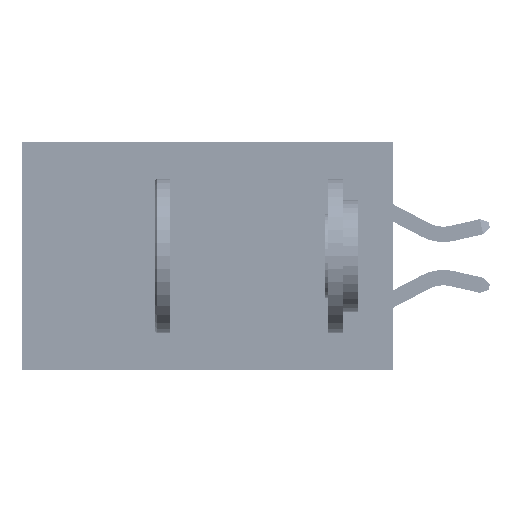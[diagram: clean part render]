
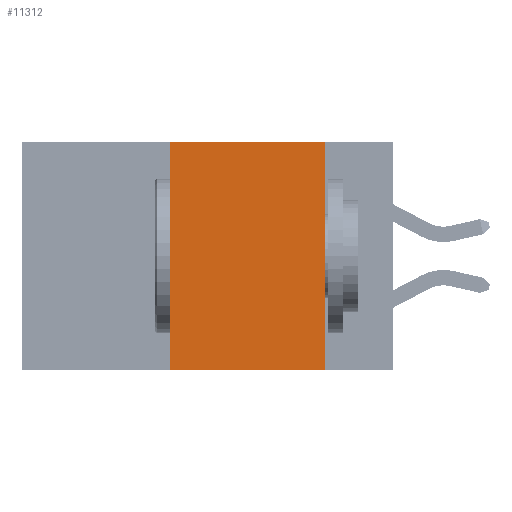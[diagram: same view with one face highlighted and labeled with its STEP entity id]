
A CAD part, left-side view. The second image highlights one B-rep face of the part: STEP entity #11312.
In plain terms, the highlighted planar face has unit normal (-1, 0, 0).
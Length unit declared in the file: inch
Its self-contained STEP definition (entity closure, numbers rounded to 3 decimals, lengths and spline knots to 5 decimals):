
#204 = FACE_OUTER_BOUND ( 'NONE', #42144, .T. ) ;
#1945 = VERTEX_POINT ( 'NONE', #15128 ) ;
#3687 = EDGE_CURVE ( 'NONE', #16818, #43986, #29375, .T. ) ;
#4079 = DIRECTION ( 'NONE',  ( 1., 0., 0. ) ) ;
#8083 = AXIS2_PLACEMENT_3D ( 'NONE', #42821, #4079, #28879 ) ;
#8617 = VECTOR ( 'NONE', #16722, 39.37008 ) ;
#10317 = DIRECTION ( 'NONE',  ( 0., 0., 1. ) ) ;
#11312 = ADVANCED_FACE ( 'NONE', ( #204 ), #25348, .F. ) ;
#11529 = ORIENTED_EDGE ( 'NONE', *, *, #35160, .T. ) ;
#12072 = CARTESIAN_POINT ( 'NONE',  ( 0., 0.36, 0. ) ) ;
#12078 = LINE ( 'NONE', #41416, #39032 ) ;
#15128 = CARTESIAN_POINT ( 'NONE',  ( 0., 0.36, -0.37 ) ) ;
#16722 = DIRECTION ( 'NONE',  ( 0., -1., 0. ) ) ;
#16818 = VERTEX_POINT ( 'NONE', #12072 ) ;
#20365 = DIRECTION ( 'NONE',  ( 0., 0., -1. ) ) ;
#21157 = DIRECTION ( 'NONE',  ( 0., -1., 0. ) ) ;
#23649 = CARTESIAN_POINT ( 'NONE',  ( 0., 0.11, -0.37 ) ) ;
#25348 = PLANE ( 'NONE',  #8083 ) ;
#26038 = CARTESIAN_POINT ( 'NONE',  ( 0., 0.11, 0. ) ) ;
#27452 = LINE ( 'NONE', #37811, #8617 ) ;
#27948 = CARTESIAN_POINT ( 'NONE',  ( 0., 0.36, 0. ) ) ;
#28879 = DIRECTION ( 'NONE',  ( 0., 0., -1. ) ) ;
#29375 = LINE ( 'NONE', #31617, #37601 ) ;
#29599 = EDGE_CURVE ( 'NONE', #1945, #16818, #36374, .T. ) ;
#31320 = VERTEX_POINT ( 'NONE', #23649 ) ;
#31617 = CARTESIAN_POINT ( 'NONE',  ( 0., 0.6, 0. ) ) ;
#34963 = ORIENTED_EDGE ( 'NONE', *, *, #29599, .F. ) ;
#35160 = EDGE_CURVE ( 'NONE', #1945, #31320, #27452, .T. ) ;
#36374 = LINE ( 'NONE', #27948, #43507 ) ;
#37601 = VECTOR ( 'NONE', #21157, 39.37008 ) ;
#37811 = CARTESIAN_POINT ( 'NONE',  ( 0., 0.6, -0.37 ) ) ;
#39032 = VECTOR ( 'NONE', #20365, 39.37008 ) ;
#39405 = ORIENTED_EDGE ( 'NONE', *, *, #45161, .F. ) ;
#41416 = CARTESIAN_POINT ( 'NONE',  ( 0., 0.11, 0. ) ) ;
#42144 = EDGE_LOOP ( 'NONE', ( #39405, #45560, #34963, #11529 ) ) ;
#42821 = CARTESIAN_POINT ( 'NONE',  ( 0., 0.6, 0. ) ) ;
#43507 = VECTOR ( 'NONE', #10317, 39.37008 ) ;
#43986 = VERTEX_POINT ( 'NONE', #26038 ) ;
#45161 = EDGE_CURVE ( 'NONE', #43986, #31320, #12078, .T. ) ;
#45560 = ORIENTED_EDGE ( 'NONE', *, *, #3687, .F. ) ;
